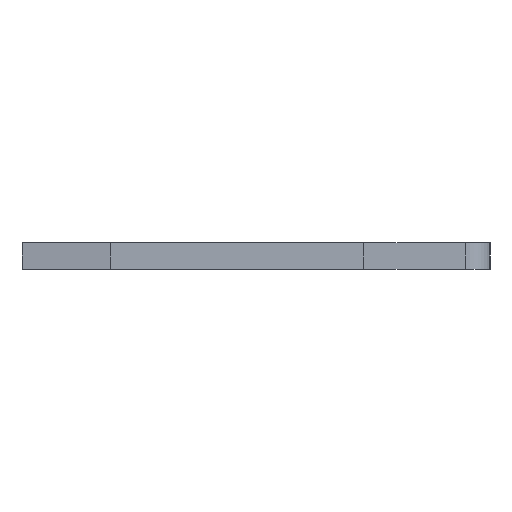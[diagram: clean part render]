
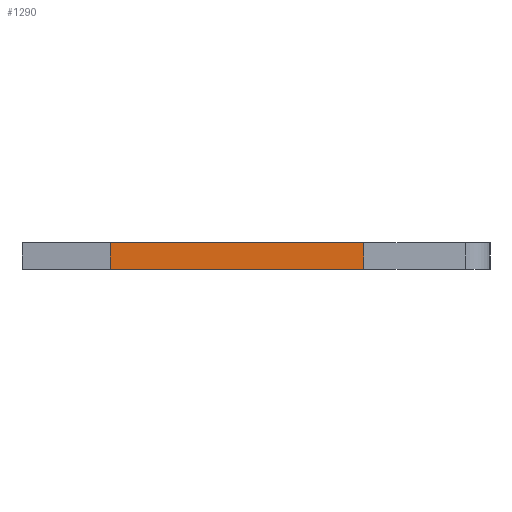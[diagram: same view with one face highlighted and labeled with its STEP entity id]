
A CAD part, left-side view. The second image highlights one B-rep face of the part: STEP entity #1290.
In plain terms, the highlighted face is planar.
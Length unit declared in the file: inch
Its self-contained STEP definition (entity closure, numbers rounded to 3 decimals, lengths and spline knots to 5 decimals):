
#61 = LINE ( 'NONE', #561, #859 ) ;
#64 = CARTESIAN_POINT ( 'NONE',  ( 0.013, 0.146, -0.0575 ) ) ;
#65 = VERTEX_POINT ( 'NONE', #1162 ) ;
#72 = EDGE_CURVE ( 'NONE', #495, #65, #323, .T. ) ;
#98 = PLANE ( 'NONE',  #705 ) ;
#163 = VERTEX_POINT ( 'NONE', #1267 ) ;
#182 = CARTESIAN_POINT ( 'NONE',  ( 0.013, 0.146, -0.0575 ) ) ;
#218 = DIRECTION ( 'NONE',  ( 0., 0., 1. ) ) ;
#245 = DIRECTION ( 'NONE',  ( -1., 0., 0. ) ) ;
#275 = VERTEX_POINT ( 'NONE', #380 ) ;
#279 = LINE ( 'NONE', #64, #1163 ) ;
#323 = LINE ( 'NONE', #1075, #1205 ) ;
#344 = EDGE_CURVE ( 'NONE', #163, #495, #279, .T. ) ;
#353 = LINE ( 'NONE', #435, #1103 ) ;
#380 = CARTESIAN_POINT ( 'NONE',  ( -0.013, -0.099, -0.0575 ) ) ;
#408 = ORIENTED_EDGE ( 'NONE', *, *, #905, .T. ) ;
#435 = CARTESIAN_POINT ( 'NONE',  ( -0.013, 0.146, -0.0575 ) ) ;
#479 = DIRECTION ( 'NONE',  ( 0., 1., 0. ) ) ;
#495 = VERTEX_POINT ( 'NONE', #182 ) ;
#520 = CARTESIAN_POINT ( 'NONE',  ( 0.013, 0.146, -0.0575 ) ) ;
#535 = DIRECTION ( 'NONE',  ( 0., 1., 0. ) ) ;
#561 = CARTESIAN_POINT ( 'NONE',  ( 0.013, -0.099, -0.0575 ) ) ;
#696 = ORIENTED_EDGE ( 'NONE', *, *, #767, .T. ) ;
#705 = AXIS2_PLACEMENT_3D ( 'NONE', #520, #218, #951 ) ;
#767 = EDGE_CURVE ( 'NONE', #275, #65, #353, .T. ) ;
#787 = DIRECTION ( 'NONE',  ( -1., 0., 0. ) ) ;
#859 = VECTOR ( 'NONE', #245, 39.37008 ) ;
#905 = EDGE_CURVE ( 'NONE', #163, #275, #61, .T. ) ;
#951 = DIRECTION ( 'NONE',  ( 1., 0., 0. ) ) ;
#1075 = CARTESIAN_POINT ( 'NONE',  ( 0.013, 0.146, -0.0575 ) ) ;
#1103 = VECTOR ( 'NONE', #535, 39.37008 ) ;
#1117 = FACE_OUTER_BOUND ( 'NONE', #1251, .T. ) ;
#1139 = ORIENTED_EDGE ( 'NONE', *, *, #72, .F. ) ;
#1154 = ORIENTED_EDGE ( 'NONE', *, *, #344, .F. ) ;
#1162 = CARTESIAN_POINT ( 'NONE',  ( -0.013, 0.146, -0.0575 ) ) ;
#1163 = VECTOR ( 'NONE', #479, 39.37008 ) ;
#1205 = VECTOR ( 'NONE', #787, 39.37008 ) ;
#1251 = EDGE_LOOP ( 'NONE', ( #696, #1139, #1154, #408 ) ) ;
#1267 = CARTESIAN_POINT ( 'NONE',  ( 0.013, -0.099, -0.0575 ) ) ;
#1290 = ADVANCED_FACE ( 'NONE', ( #1117 ), #98, .F. ) ;
